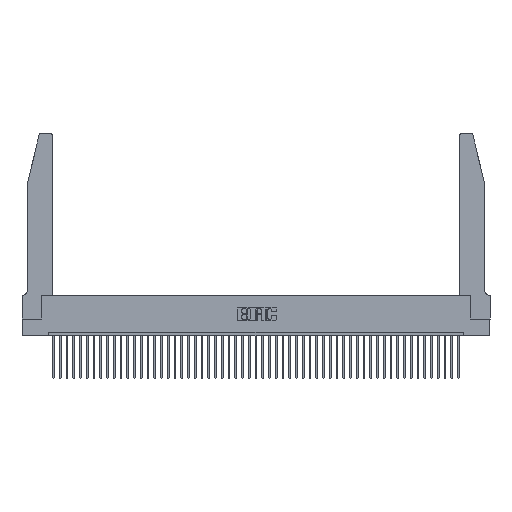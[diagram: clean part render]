
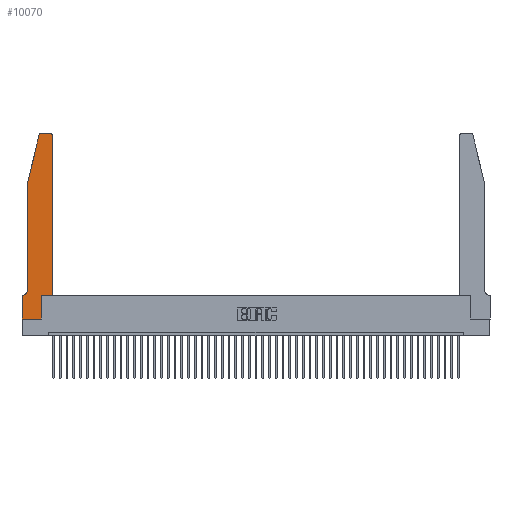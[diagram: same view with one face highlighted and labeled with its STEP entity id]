
A CAD part, top view. The second image highlights one B-rep face of the part: STEP entity #10070.
In plain terms, the highlighted planar face has unit normal (0, 0, 1).
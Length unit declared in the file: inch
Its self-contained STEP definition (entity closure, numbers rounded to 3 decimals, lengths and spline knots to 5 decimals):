
#986 = CARTESIAN_POINT ( 'NONE',  ( 0.2865, 0.35, 0.37 ) ) ;
#1673 = AXIS2_PLACEMENT_3D ( 'NONE', #40227, #11136, #43691 ) ;
#2187 = ORIENTED_EDGE ( 'NONE', *, *, #31792, .T. ) ;
#3228 = EDGE_CURVE ( 'NONE', #17947, #17634, #37606, .T. ) ;
#3268 = CARTESIAN_POINT ( 'NONE',  ( 0.0755, 2., 0.37 ) ) ;
#3306 = EDGE_CURVE ( 'NONE', #27154, #36722, #38119, .T. ) ;
#4283 = CARTESIAN_POINT ( 'NONE',  ( 0.4505, 0.35, 0.37 ) ) ;
#4411 = CARTESIAN_POINT ( 'NONE',  ( 0.284, 2.72, 0.37 ) ) ;
#5027 = CARTESIAN_POINT ( 'NONE',  ( 0.4505, 0.35, 0.37 ) ) ;
#5580 = CIRCLE ( 'NONE', #7276, 0.03 ) ;
#6824 = DIRECTION ( 'NONE',  ( 0., 0., 1. ) ) ;
#7276 = AXIS2_PLACEMENT_3D ( 'NONE', #44170, #6824, #36852 ) ;
#7440 = CARTESIAN_POINT ( 'NONE',  ( 0., 0., 0.37 ) ) ;
#8029 = DIRECTION ( 'NONE',  ( 1., 0., 0. ) ) ;
#8659 = CIRCLE ( 'NONE', #40231, 0.07 ) ;
#9201 = ORIENTED_EDGE ( 'NONE', *, *, #34428, .T. ) ;
#10070 = ADVANCED_FACE ( 'NONE', ( #33422 ), #29007, .T. ) ;
#10260 = CARTESIAN_POINT ( 'NONE',  ( 0.0755, 0.42, 0.37 ) ) ;
#10459 = LINE ( 'NONE', #4283, #33052 ) ;
#11136 = DIRECTION ( 'NONE',  ( 0., 0., 1. ) ) ;
#11575 = VERTEX_POINT ( 'NONE', #36408 ) ;
#11608 = VERTEX_POINT ( 'NONE', #25631 ) ;
#12139 = DIRECTION ( 'NONE',  ( -0.239, -0.971, 0. ) ) ;
#12443 = VECTOR ( 'NONE', #12139, 39.37008 ) ;
#12964 = EDGE_CURVE ( 'NONE', #17634, #33903, #35517, .T. ) ;
#13118 = DIRECTION ( 'NONE',  ( 0., -1., 0. ) ) ;
#13307 = VERTEX_POINT ( 'NONE', #43947 ) ;
#14145 = VERTEX_POINT ( 'NONE', #10260 ) ;
#14646 = EDGE_CURVE ( 'NONE', #13307, #11575, #15991, .T. ) ;
#15612 = CARTESIAN_POINT ( 'NONE',  ( 0.0055, 0.42, 0.37 ) ) ;
#15991 = LINE ( 'NONE', #30527, #16599 ) ;
#16170 = EDGE_CURVE ( 'NONE', #27612, #29963, #39223, .T. ) ;
#16259 = LINE ( 'NONE', #39573, #32580 ) ;
#16509 = CARTESIAN_POINT ( 'NONE',  ( 0.0055, 0.35, 0.37 ) ) ;
#16599 = VECTOR ( 'NONE', #38680, 39.37008 ) ;
#17308 = AXIS2_PLACEMENT_3D ( 'NONE', #4411, #22910, #8029 ) ;
#17634 = VERTEX_POINT ( 'NONE', #30305 ) ;
#17812 = VECTOR ( 'NONE', #21952, 39.37008 ) ;
#17947 = VERTEX_POINT ( 'NONE', #32775 ) ;
#18798 = CARTESIAN_POINT ( 'NONE',  ( 0.0755, 0.35, 0.37 ) ) ;
#19317 = DIRECTION ( 'NONE',  ( 0., 0., -1. ) ) ;
#20062 = VECTOR ( 'NONE', #40797, 39.37008 ) ;
#21149 = DIRECTION ( 'NONE',  ( 0., 1., 0. ) ) ;
#21952 = DIRECTION ( 'NONE',  ( 1., 0., 0. ) ) ;
#22542 = ORIENTED_EDGE ( 'NONE', *, *, #25624, .T. ) ;
#22910 = DIRECTION ( 'NONE',  ( 0., 0., 1. ) ) ;
#22927 = ORIENTED_EDGE ( 'NONE', *, *, #42540, .T. ) ;
#25001 = EDGE_CURVE ( 'NONE', #11575, #27612, #47045, .T. ) ;
#25229 = EDGE_CURVE ( 'NONE', #36722, #17947, #37102, .T. ) ;
#25624 = EDGE_CURVE ( 'NONE', #33903, #26071, #36543, .T. ) ;
#25631 = CARTESIAN_POINT ( 'NONE',  ( 0.4505, 2.72, 0.37 ) ) ;
#26071 = VERTEX_POINT ( 'NONE', #5027 ) ;
#27154 = VERTEX_POINT ( 'NONE', #16509 ) ;
#27612 = VERTEX_POINT ( 'NONE', #39482 ) ;
#28116 = ORIENTED_EDGE ( 'NONE', *, *, #12964, .T. ) ;
#28250 = ORIENTED_EDGE ( 'NONE', *, *, #16170, .T. ) ;
#28974 = VECTOR ( 'NONE', #32377, 39.37008 ) ;
#29007 = PLANE ( 'NONE',  #1673 ) ;
#29018 = VECTOR ( 'NONE', #40591, 39.37008 ) ;
#29963 = VERTEX_POINT ( 'NONE', #3268 ) ;
#30305 = CARTESIAN_POINT ( 'NONE',  ( 0.2865, 0., 0.37 ) ) ;
#30527 = CARTESIAN_POINT ( 'NONE',  ( 0.2605, 2.75, 0.37 ) ) ;
#30603 = ORIENTED_EDGE ( 'NONE', *, *, #14646, .T. ) ;
#30656 = CARTESIAN_POINT ( 'NONE',  ( 0.0755, 2., 0.37 ) ) ;
#31668 = ORIENTED_EDGE ( 'NONE', *, *, #25001, .T. ) ;
#31792 = EDGE_CURVE ( 'NONE', #29963, #14145, #16259, .T. ) ;
#32377 = DIRECTION ( 'NONE',  ( 1., 0., 0. ) ) ;
#32414 = ORIENTED_EDGE ( 'NONE', *, *, #25229, .T. ) ;
#32580 = VECTOR ( 'NONE', #13118, 39.37008 ) ;
#32775 = CARTESIAN_POINT ( 'NONE',  ( 0., 0., 0.37 ) ) ;
#32974 = ORIENTED_EDGE ( 'NONE', *, *, #3306, .T. ) ;
#33052 = VECTOR ( 'NONE', #41060, 39.37008 ) ;
#33422 = FACE_OUTER_BOUND ( 'NONE', #46660, .T. ) ;
#33903 = VERTEX_POINT ( 'NONE', #986 ) ;
#34324 = VECTOR ( 'NONE', #21149, 39.37008 ) ;
#34428 = EDGE_CURVE ( 'NONE', #11608, #13307, #5580, .T. ) ;
#34812 = CARTESIAN_POINT ( 'NONE',  ( 0.4505, 0.35, 0.37 ) ) ;
#35517 = LINE ( 'NONE', #38412, #34324 ) ;
#36408 = CARTESIAN_POINT ( 'NONE',  ( 0.284, 2.75, 0.37 ) ) ;
#36543 = LINE ( 'NONE', #34812, #28974 ) ;
#36722 = VERTEX_POINT ( 'NONE', #38706 ) ;
#36852 = DIRECTION ( 'NONE',  ( 1., 0., 0. ) ) ;
#37102 = LINE ( 'NONE', #7440, #29018 ) ;
#37606 = LINE ( 'NONE', #40684, #17812 ) ;
#38119 = LINE ( 'NONE', #18798, #20062 ) ;
#38412 = CARTESIAN_POINT ( 'NONE',  ( 0.2865, 0.35, 0.37 ) ) ;
#38680 = DIRECTION ( 'NONE',  ( -1., 0., 0. ) ) ;
#38706 = CARTESIAN_POINT ( 'NONE',  ( 0., 0.35, 0.37 ) ) ;
#39223 = LINE ( 'NONE', #30656, #12443 ) ;
#39482 = CARTESIAN_POINT ( 'NONE',  ( 0.25487, 2.72718, 0.37 ) ) ;
#39573 = CARTESIAN_POINT ( 'NONE',  ( 0.0755, 2., 0.37 ) ) ;
#40227 = CARTESIAN_POINT ( 'NONE',  ( 0., 0.35, 0.37 ) ) ;
#40231 = AXIS2_PLACEMENT_3D ( 'NONE', #15612, #19317, #45050 ) ;
#40591 = DIRECTION ( 'NONE',  ( 0., -1., 0. ) ) ;
#40684 = CARTESIAN_POINT ( 'NONE',  ( 0., 0., 0.37 ) ) ;
#40797 = DIRECTION ( 'NONE',  ( -1., 0., 0. ) ) ;
#41060 = DIRECTION ( 'NONE',  ( 0., 1., 0. ) ) ;
#42540 = EDGE_CURVE ( 'NONE', #26071, #11608, #10459, .T. ) ;
#43180 = EDGE_CURVE ( 'NONE', #14145, #27154, #8659, .T. ) ;
#43691 = DIRECTION ( 'NONE',  ( 1., 0., 0. ) ) ;
#43947 = CARTESIAN_POINT ( 'NONE',  ( 0.4205, 2.75, 0.37 ) ) ;
#44170 = CARTESIAN_POINT ( 'NONE',  ( 0.4205, 2.72, 0.37 ) ) ;
#45050 = DIRECTION ( 'NONE',  ( -1., 0., 0. ) ) ;
#46154 = ORIENTED_EDGE ( 'NONE', *, *, #43180, .T. ) ;
#46199 = ORIENTED_EDGE ( 'NONE', *, *, #3228, .T. ) ;
#46660 = EDGE_LOOP ( 'NONE', ( #30603, #31668, #28250, #2187, #46154, #32974, #32414, #46199, #28116, #22542, #22927, #9201 ) ) ;
#47045 = CIRCLE ( 'NONE', #17308, 0.03 ) ;
